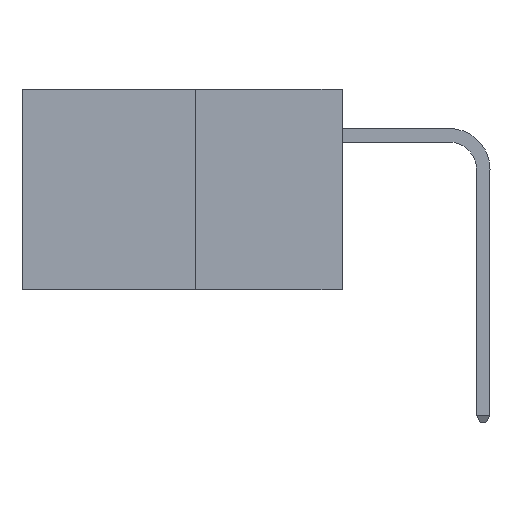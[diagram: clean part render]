
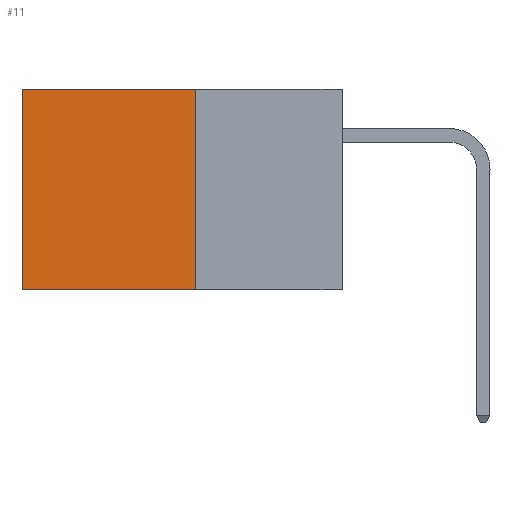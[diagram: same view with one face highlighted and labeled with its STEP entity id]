
A CAD part, left-side view. The second image highlights one B-rep face of the part: STEP entity #11.
In plain terms, the highlighted planar face has unit normal (-1, 0, 0).
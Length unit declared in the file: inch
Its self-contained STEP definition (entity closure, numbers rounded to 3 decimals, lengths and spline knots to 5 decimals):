
#11 = ADVANCED_FACE ( 'NONE', ( #6908 ), #5823, .F. ) ;
#622 = VECTOR ( 'NONE', #13641, 39.37008 ) ;
#854 = ORIENTED_EDGE ( 'NONE', *, *, #17109, .T. ) ;
#1895 = CARTESIAN_POINT ( 'NONE',  ( 0.277, 0.59, 0. ) ) ;
#3534 = LINE ( 'NONE', #10683, #7361 ) ;
#3549 = EDGE_LOOP ( 'NONE', ( #16608, #13883, #11897, #854 ) ) ;
#3793 = AXIS2_PLACEMENT_3D ( 'NONE', #9190, #13573, #13255 ) ;
#4165 = CARTESIAN_POINT ( 'NONE',  ( 0.277, 0.59, -0.37 ) ) ;
#4199 = EDGE_CURVE ( 'NONE', #11506, #14096, #11888, .T. ) ;
#5823 = PLANE ( 'NONE',  #3793 ) ;
#6908 = FACE_OUTER_BOUND ( 'NONE', #3549, .T. ) ;
#7058 = DIRECTION ( 'NONE',  ( 0., 0., -1. ) ) ;
#7361 = VECTOR ( 'NONE', #8027, 39.37008 ) ;
#7994 = CARTESIAN_POINT ( 'NONE',  ( 0.277, 0.27, -0.37 ) ) ;
#8027 = DIRECTION ( 'NONE',  ( 0., 1., 0. ) ) ;
#8746 = EDGE_CURVE ( 'NONE', #10307, #14525, #9622, .T. ) ;
#9190 = CARTESIAN_POINT ( 'NONE',  ( 0.277, 0.27, -0.37 ) ) ;
#9198 = VECTOR ( 'NONE', #7058, 39.37008 ) ;
#9278 = LINE ( 'NONE', #7994, #15774 ) ;
#9622 = LINE ( 'NONE', #4165, #9198 ) ;
#10307 = VERTEX_POINT ( 'NONE', #1895 ) ;
#10683 = CARTESIAN_POINT ( 'NONE',  ( 0.277, 0.27, 0. ) ) ;
#10712 = DIRECTION ( 'NONE',  ( 0., 1., 0. ) ) ;
#11506 = VERTEX_POINT ( 'NONE', #17622 ) ;
#11888 = LINE ( 'NONE', #12364, #622 ) ;
#11897 = ORIENTED_EDGE ( 'NONE', *, *, #4199, .F. ) ;
#12364 = CARTESIAN_POINT ( 'NONE',  ( 0.277, 0.27, -0.37 ) ) ;
#13255 = DIRECTION ( 'NONE',  ( 0., 0., -1. ) ) ;
#13406 = CARTESIAN_POINT ( 'NONE',  ( 0.277, 0.27, -0.37 ) ) ;
#13573 = DIRECTION ( 'NONE',  ( 1., 0., 0. ) ) ;
#13641 = DIRECTION ( 'NONE',  ( 0., 0., -1. ) ) ;
#13883 = ORIENTED_EDGE ( 'NONE', *, *, #15290, .F. ) ;
#14096 = VERTEX_POINT ( 'NONE', #13406 ) ;
#14510 = CARTESIAN_POINT ( 'NONE',  ( 0.277, 0.59, -0.37 ) ) ;
#14525 = VERTEX_POINT ( 'NONE', #14510 ) ;
#15290 = EDGE_CURVE ( 'NONE', #14096, #14525, #9278, .T. ) ;
#15774 = VECTOR ( 'NONE', #10712, 39.37008 ) ;
#16608 = ORIENTED_EDGE ( 'NONE', *, *, #8746, .T. ) ;
#17109 = EDGE_CURVE ( 'NONE', #11506, #10307, #3534, .T. ) ;
#17622 = CARTESIAN_POINT ( 'NONE',  ( 0.277, 0.27, 0. ) ) ;
